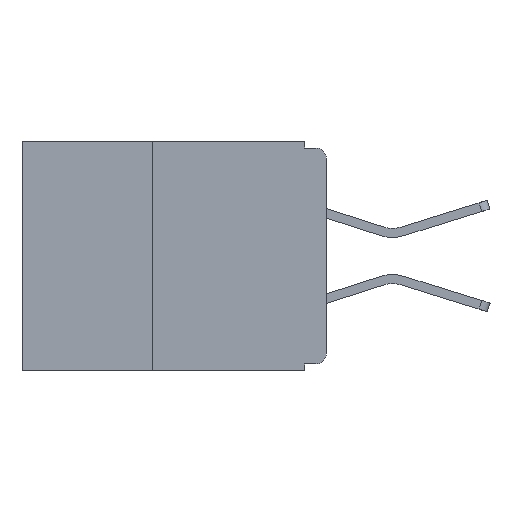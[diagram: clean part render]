
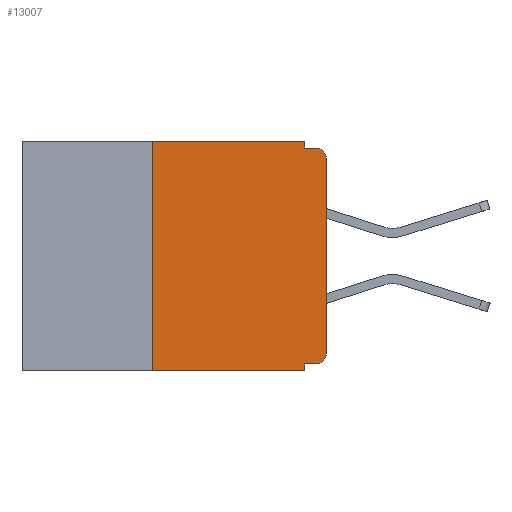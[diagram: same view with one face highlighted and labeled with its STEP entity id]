
A CAD part, left-side view. The second image highlights one B-rep face of the part: STEP entity #13007.
In plain terms, the highlighted planar face has unit normal (-1, 0, 0).
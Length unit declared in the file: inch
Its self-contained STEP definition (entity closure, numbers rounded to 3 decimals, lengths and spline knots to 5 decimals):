
#114 = CARTESIAN_POINT ( 'NONE',  ( 0., 0.031, -0.01 ) ) ;
#284 = VECTOR ( 'NONE', #16698, 39.37008 ) ;
#584 = LINE ( 'NONE', #18240, #15590 ) ;
#878 = CARTESIAN_POINT ( 'NONE',  ( 0., 0., 0. ) ) ;
#1214 = VERTEX_POINT ( 'NONE', #114 ) ;
#1933 = ORIENTED_EDGE ( 'NONE', *, *, #9804, .T. ) ;
#2026 = EDGE_CURVE ( 'NONE', #3888, #16474, #11717, .T. ) ;
#2146 = ORIENTED_EDGE ( 'NONE', *, *, #9722, .T. ) ;
#2508 = EDGE_CURVE ( 'NONE', #1214, #4663, #584, .T. ) ;
#2512 = DIRECTION ( 'NONE',  ( 0., 0., -1. ) ) ;
#2554 = LINE ( 'NONE', #878, #9551 ) ;
#2856 = ORIENTED_EDGE ( 'NONE', *, *, #2508, .F. ) ;
#3049 = LINE ( 'NONE', #13505, #7074 ) ;
#3143 = FACE_OUTER_BOUND ( 'NONE', #12512, .T. ) ;
#3261 = CARTESIAN_POINT ( 'NONE',  ( 0., 0.031, -0.33 ) ) ;
#3346 = DIRECTION ( 'NONE',  ( 0., 1., 0. ) ) ;
#3350 = VERTEX_POINT ( 'NONE', #16210 ) ;
#3713 = ORIENTED_EDGE ( 'NONE', *, *, #4193, .F. ) ;
#3802 = ORIENTED_EDGE ( 'NONE', *, *, #13855, .F. ) ;
#3888 = VERTEX_POINT ( 'NONE', #5713 ) ;
#4193 = EDGE_CURVE ( 'NONE', #8917, #1214, #12119, .T. ) ;
#4207 = CARTESIAN_POINT ( 'NONE',  ( 0., 0.25, -0.33 ) ) ;
#4232 = VECTOR ( 'NONE', #13342, 39.37008 ) ;
#4287 = ORIENTED_EDGE ( 'NONE', *, *, #9900, .F. ) ;
#4423 = ORIENTED_EDGE ( 'NONE', *, *, #6137, .T. ) ;
#4663 = VERTEX_POINT ( 'NONE', #10016 ) ;
#5571 = CARTESIAN_POINT ( 'NONE',  ( 0., 0.031, -0.33 ) ) ;
#5713 = CARTESIAN_POINT ( 'NONE',  ( 0., 0.031, -0.32 ) ) ;
#6137 = EDGE_CURVE ( 'NONE', #16229, #16474, #7132, .T. ) ;
#6444 = VERTEX_POINT ( 'NONE', #7888 ) ;
#6517 = ORIENTED_EDGE ( 'NONE', *, *, #2026, .F. ) ;
#7058 = DIRECTION ( 'NONE',  ( 0., 0., -1. ) ) ;
#7074 = VECTOR ( 'NONE', #3346, 39.37008 ) ;
#7076 = DIRECTION ( 'NONE',  ( -1., 0., 0. ) ) ;
#7095 = CARTESIAN_POINT ( 'NONE',  ( 0., 0.015, -0.305 ) ) ;
#7132 = LINE ( 'NONE', #14399, #14216 ) ;
#7597 = ORIENTED_EDGE ( 'NONE', *, *, #15899, .F. ) ;
#7678 = CARTESIAN_POINT ( 'NONE',  ( 0., 0.031, 0. ) ) ;
#7816 = DIRECTION ( 'NONE',  ( 0., -1., 0. ) ) ;
#7888 = CARTESIAN_POINT ( 'NONE',  ( 0., 0.25, 0. ) ) ;
#8034 = AXIS2_PLACEMENT_3D ( 'NONE', #17624, #17498, #17463 ) ;
#8090 = CARTESIAN_POINT ( 'NONE',  ( 0., 0., -0.305 ) ) ;
#8207 = LINE ( 'NONE', #12719, #4232 ) ;
#8917 = VERTEX_POINT ( 'NONE', #7678 ) ;
#8969 = ORIENTED_EDGE ( 'NONE', *, *, #14176, .T. ) ;
#9235 = AXIS2_PLACEMENT_3D ( 'NONE', #11204, #10824, #10392 ) ;
#9551 = VECTOR ( 'NONE', #18669, 39.37008 ) ;
#9722 = EDGE_CURVE ( 'NONE', #16113, #4663, #11353, .T. ) ;
#9804 = EDGE_CURVE ( 'NONE', #11245, #16113, #2554, .T. ) ;
#9900 = EDGE_CURVE ( 'NONE', #16229, #6444, #8207, .T. ) ;
#10016 = CARTESIAN_POINT ( 'NONE',  ( 0., 0.015, -0.01 ) ) ;
#10176 = DIRECTION ( 'NONE',  ( 0., -1., 0. ) ) ;
#10238 = CARTESIAN_POINT ( 'NONE',  ( 0., 0.437, 0. ) ) ;
#10392 = DIRECTION ( 'NONE',  ( 0., 0., -1. ) ) ;
#10437 = AXIS2_PLACEMENT_3D ( 'NONE', #7095, #7076, #7058 ) ;
#10824 = DIRECTION ( 'NONE',  ( -1., 0., 0. ) ) ;
#11204 = CARTESIAN_POINT ( 'NONE',  ( 0., 0.015, -0.025 ) ) ;
#11245 = VERTEX_POINT ( 'NONE', #8090 ) ;
#11353 = CIRCLE ( 'NONE', #9235, 0.015 ) ;
#11717 = LINE ( 'NONE', #5571, #15341 ) ;
#12119 = LINE ( 'NONE', #16695, #284 ) ;
#12512 = EDGE_LOOP ( 'NONE', ( #1933, #2146, #2856, #3713, #3802, #4287, #4423, #6517, #7597, #8969 ) ) ;
#12699 = CIRCLE ( 'NONE', #10437, 0.015 ) ;
#12719 = CARTESIAN_POINT ( 'NONE',  ( 0., 0.25, -0.33 ) ) ;
#13007 = ADVANCED_FACE ( 'NONE', ( #3143 ), #17731, .F. ) ;
#13342 = DIRECTION ( 'NONE',  ( 0., 0., 1. ) ) ;
#13505 = CARTESIAN_POINT ( 'NONE',  ( 0., 0., -0.32 ) ) ;
#13855 = EDGE_CURVE ( 'NONE', #6444, #8917, #15769, .T. ) ;
#14176 = EDGE_CURVE ( 'NONE', #3350, #11245, #12699, .T. ) ;
#14201 = DIRECTION ( 'NONE',  ( 0., -1., 0. ) ) ;
#14216 = VECTOR ( 'NONE', #14201, 39.37008 ) ;
#14399 = CARTESIAN_POINT ( 'NONE',  ( 0., 0.437, -0.33 ) ) ;
#15341 = VECTOR ( 'NONE', #2512, 39.37008 ) ;
#15590 = VECTOR ( 'NONE', #7816, 39.37008 ) ;
#15769 = LINE ( 'NONE', #10238, #18271 ) ;
#15899 = EDGE_CURVE ( 'NONE', #3350, #3888, #3049, .T. ) ;
#16113 = VERTEX_POINT ( 'NONE', #18051 ) ;
#16210 = CARTESIAN_POINT ( 'NONE',  ( 0., 0.015, -0.32 ) ) ;
#16229 = VERTEX_POINT ( 'NONE', #4207 ) ;
#16474 = VERTEX_POINT ( 'NONE', #3261 ) ;
#16695 = CARTESIAN_POINT ( 'NONE',  ( 0., 0.031, 0. ) ) ;
#16698 = DIRECTION ( 'NONE',  ( 0., 0., -1. ) ) ;
#17463 = DIRECTION ( 'NONE',  ( 0., 0., -1. ) ) ;
#17498 = DIRECTION ( 'NONE',  ( 1., 0., 0. ) ) ;
#17624 = CARTESIAN_POINT ( 'NONE',  ( 0., 0.437, 0. ) ) ;
#17731 = PLANE ( 'NONE',  #8034 ) ;
#18051 = CARTESIAN_POINT ( 'NONE',  ( 0., 0., -0.025 ) ) ;
#18240 = CARTESIAN_POINT ( 'NONE',  ( 0., 0., -0.01 ) ) ;
#18271 = VECTOR ( 'NONE', #10176, 39.37008 ) ;
#18669 = DIRECTION ( 'NONE',  ( 0., 0., 1. ) ) ;
